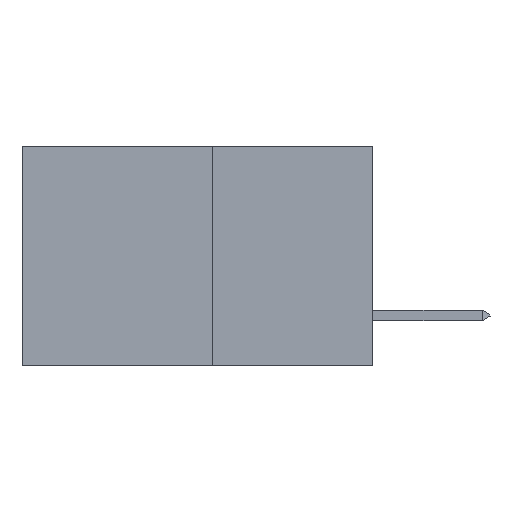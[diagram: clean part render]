
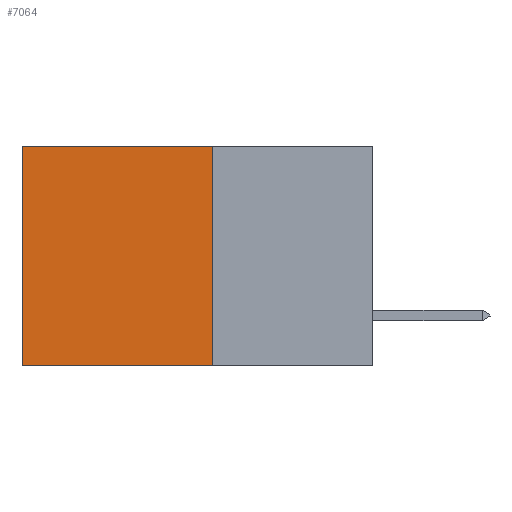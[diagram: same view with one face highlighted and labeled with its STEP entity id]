
A CAD part, left-side view. The second image highlights one B-rep face of the part: STEP entity #7064.
In plain terms, the highlighted planar face has unit normal (-1, 0, 0).
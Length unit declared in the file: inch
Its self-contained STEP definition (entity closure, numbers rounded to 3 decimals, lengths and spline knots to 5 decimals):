
#8 = CARTESIAN_POINT ( 'NONE',  ( 0.277, 0.27, -0.37 ) ) ;
#205 = AXIS2_PLACEMENT_3D ( 'NONE', #2869, #2795, #2654 ) ;
#392 = LINE ( 'NONE', #1078, #8252 ) ;
#1078 = CARTESIAN_POINT ( 'NONE',  ( 0.277, 0.59, -0.37 ) ) ;
#1311 = DIRECTION ( 'NONE',  ( 0., 0., -1. ) ) ;
#2654 = DIRECTION ( 'NONE',  ( 0., 0., -1. ) ) ;
#2795 = DIRECTION ( 'NONE',  ( 1., 0., 0. ) ) ;
#2869 = CARTESIAN_POINT ( 'NONE',  ( 0.277, 0.27, -0.37 ) ) ;
#2912 = VERTEX_POINT ( 'NONE', #3996 ) ;
#2977 = LINE ( 'NONE', #4792, #13614 ) ;
#3427 = PLANE ( 'NONE',  #205 ) ;
#3462 = VERTEX_POINT ( 'NONE', #5363 ) ;
#3615 = CARTESIAN_POINT ( 'NONE',  ( 0.277, 0.27, 0. ) ) ;
#3670 = FACE_OUTER_BOUND ( 'NONE', #4591, .T. ) ;
#3996 = CARTESIAN_POINT ( 'NONE',  ( 0.277, 0.27, -0.37 ) ) ;
#4591 = EDGE_LOOP ( 'NONE', ( #5253, #8358, #10670, #8886 ) ) ;
#4792 = CARTESIAN_POINT ( 'NONE',  ( 0.277, 0.27, 0. ) ) ;
#5168 = EDGE_CURVE ( 'NONE', #2912, #8523, #10472, .T. ) ;
#5187 = EDGE_CURVE ( 'NONE', #9682, #2912, #12485, .T. ) ;
#5253 = ORIENTED_EDGE ( 'NONE', *, *, #7131, .T. ) ;
#5363 = CARTESIAN_POINT ( 'NONE',  ( 0.277, 0.59, 0. ) ) ;
#6630 = CARTESIAN_POINT ( 'NONE',  ( 0.277, 0.27, -0.37 ) ) ;
#6701 = DIRECTION ( 'NONE',  ( 0., 1., 0. ) ) ;
#7064 = ADVANCED_FACE ( 'NONE', ( #3670 ), #3427, .F. ) ;
#7131 = EDGE_CURVE ( 'NONE', #3462, #8523, #392, .T. ) ;
#7652 = VECTOR ( 'NONE', #13615, 39.37008 ) ;
#8252 = VECTOR ( 'NONE', #1311, 39.37008 ) ;
#8358 = ORIENTED_EDGE ( 'NONE', *, *, #5168, .F. ) ;
#8523 = VERTEX_POINT ( 'NONE', #9457 ) ;
#8886 = ORIENTED_EDGE ( 'NONE', *, *, #8958, .T. ) ;
#8958 = EDGE_CURVE ( 'NONE', #9682, #3462, #2977, .T. ) ;
#9014 = DIRECTION ( 'NONE',  ( 0., 1., 0. ) ) ;
#9457 = CARTESIAN_POINT ( 'NONE',  ( 0.277, 0.59, -0.37 ) ) ;
#9682 = VERTEX_POINT ( 'NONE', #3615 ) ;
#10174 = VECTOR ( 'NONE', #6701, 39.37008 ) ;
#10472 = LINE ( 'NONE', #6630, #10174 ) ;
#10670 = ORIENTED_EDGE ( 'NONE', *, *, #5187, .F. ) ;
#12485 = LINE ( 'NONE', #8, #7652 ) ;
#13614 = VECTOR ( 'NONE', #9014, 39.37008 ) ;
#13615 = DIRECTION ( 'NONE',  ( 0., 0., -1. ) ) ;
